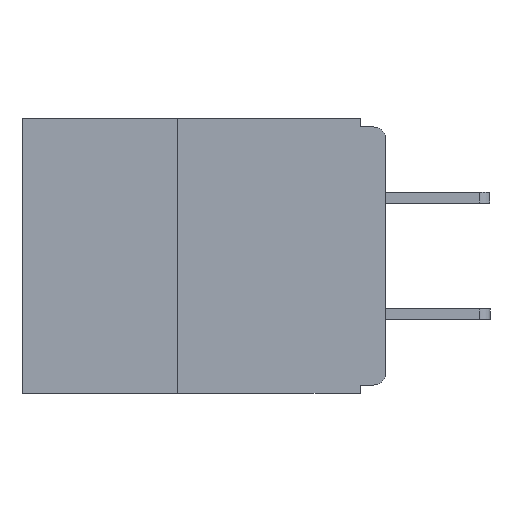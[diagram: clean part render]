
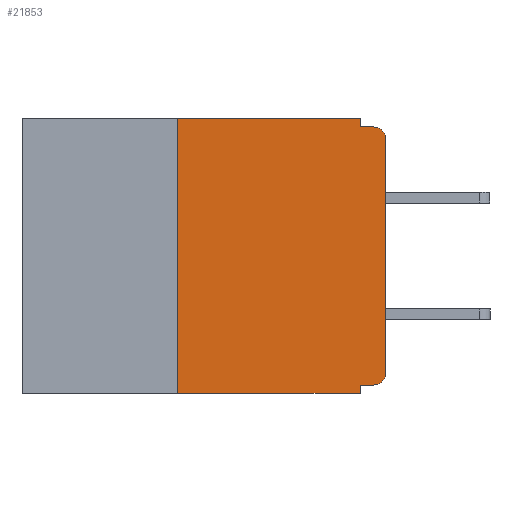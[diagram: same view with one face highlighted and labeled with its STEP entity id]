
A CAD part, left-side view. The second image highlights one B-rep face of the part: STEP entity #21853.
In plain terms, the highlighted planar face has unit normal (-1, 0, 0).
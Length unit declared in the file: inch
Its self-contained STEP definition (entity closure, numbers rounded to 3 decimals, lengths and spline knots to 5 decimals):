
#26 = DIRECTION ( 'NONE',  ( 0., 0., -1. ) ) ;
#182 = LINE ( 'NONE', #5568, #24632 ) ;
#545 = CIRCLE ( 'NONE', #4228, 0.015 ) ;
#1150 = VERTEX_POINT ( 'NONE', #28312 ) ;
#1469 = EDGE_CURVE ( 'NONE', #29636, #2069, #15435, .T. ) ;
#1866 = CARTESIAN_POINT ( 'NONE',  ( 0., 0.031, 0. ) ) ;
#1931 = LINE ( 'NONE', #22578, #26181 ) ;
#1976 = CARTESIAN_POINT ( 'NONE',  ( 0., 0.031, -0.33 ) ) ;
#2069 = VERTEX_POINT ( 'NONE', #25018 ) ;
#2097 = DIRECTION ( 'NONE',  ( 0., 0., -1. ) ) ;
#2190 = VECTOR ( 'NONE', #18975, 39.37008 ) ;
#2293 = VERTEX_POINT ( 'NONE', #10409 ) ;
#2491 = VECTOR ( 'NONE', #17809, 39.37008 ) ;
#2676 = FACE_OUTER_BOUND ( 'NONE', #25250, .T. ) ;
#2992 = ORIENTED_EDGE ( 'NONE', *, *, #18980, .T. ) ;
#3716 = LINE ( 'NONE', #15430, #27130 ) ;
#3831 = CARTESIAN_POINT ( 'NONE',  ( 0., 0.031, -0.01 ) ) ;
#4228 = AXIS2_PLACEMENT_3D ( 'NONE', #13681, #29791, #16025 ) ;
#5568 = CARTESIAN_POINT ( 'NONE',  ( 0., 0.031, 0. ) ) ;
#5928 = ORIENTED_EDGE ( 'NONE', *, *, #9402, .F. ) ;
#6290 = ORIENTED_EDGE ( 'NONE', *, *, #24210, .T. ) ;
#7360 = ORIENTED_EDGE ( 'NONE', *, *, #25891, .F. ) ;
#7469 = VERTEX_POINT ( 'NONE', #1866 ) ;
#8185 = DIRECTION ( 'NONE',  ( 0., 0., 1. ) ) ;
#8435 = AXIS2_PLACEMENT_3D ( 'NONE', #13948, #16298, #2097 ) ;
#8697 = LINE ( 'NONE', #24704, #2491 ) ;
#9402 = EDGE_CURVE ( 'NONE', #20168, #25844, #14808, .T. ) ;
#9534 = CARTESIAN_POINT ( 'NONE',  ( 0., 0.031, -0.33 ) ) ;
#10409 = CARTESIAN_POINT ( 'NONE',  ( 0., 0., -0.305 ) ) ;
#10412 = CARTESIAN_POINT ( 'NONE',  ( 0., 0.015, -0.01 ) ) ;
#10451 = LINE ( 'NONE', #9534, #16031 ) ;
#10753 = DIRECTION ( 'NONE',  ( 0., -1., 0. ) ) ;
#10789 = VERTEX_POINT ( 'NONE', #28320 ) ;
#11145 = ORIENTED_EDGE ( 'NONE', *, *, #1469, .F. ) ;
#12031 = CARTESIAN_POINT ( 'NONE',  ( 0., 0.015, -0.025 ) ) ;
#13215 = VERTEX_POINT ( 'NONE', #1976 ) ;
#13681 = CARTESIAN_POINT ( 'NONE',  ( 0., 0.015, -0.305 ) ) ;
#13945 = VERTEX_POINT ( 'NONE', #23616 ) ;
#13948 = CARTESIAN_POINT ( 'NONE',  ( 0., 0.437, 0. ) ) ;
#14240 = CARTESIAN_POINT ( 'NONE',  ( 0., 0., -0.01 ) ) ;
#14371 = CARTESIAN_POINT ( 'NONE',  ( 0., 0.015, -0.32 ) ) ;
#14409 = DIRECTION ( 'NONE',  ( 0., 0., -1. ) ) ;
#14808 = LINE ( 'NONE', #14240, #2190 ) ;
#15245 = ORIENTED_EDGE ( 'NONE', *, *, #21317, .F. ) ;
#15417 = CARTESIAN_POINT ( 'NONE',  ( 0., 0., -0.32 ) ) ;
#15430 = CARTESIAN_POINT ( 'NONE',  ( 0., 0.437, -0.33 ) ) ;
#15435 = LINE ( 'NONE', #15417, #20929 ) ;
#15629 = VECTOR ( 'NONE', #8185, 39.37008 ) ;
#16025 = DIRECTION ( 'NONE',  ( 0., 0., -1. ) ) ;
#16031 = VECTOR ( 'NONE', #26, 39.37008 ) ;
#16298 = DIRECTION ( 'NONE',  ( 1., 0., 0. ) ) ;
#17693 = CARTESIAN_POINT ( 'NONE',  ( 0., 0.25, -0.33 ) ) ;
#17809 = DIRECTION ( 'NONE',  ( 0., -1., 0. ) ) ;
#18975 = DIRECTION ( 'NONE',  ( 0., -1., 0. ) ) ;
#18980 = EDGE_CURVE ( 'NONE', #2293, #1150, #1931, .T. ) ;
#19727 = DIRECTION ( 'NONE',  ( 0., 0., -1. ) ) ;
#20168 = VERTEX_POINT ( 'NONE', #3831 ) ;
#20929 = VECTOR ( 'NONE', #27915, 39.37008 ) ;
#21317 = EDGE_CURVE ( 'NONE', #2069, #13215, #10451, .T. ) ;
#21853 = ADVANCED_FACE ( 'NONE', ( #2676 ), #27803, .F. ) ;
#22578 = CARTESIAN_POINT ( 'NONE',  ( 0., 0., 0. ) ) ;
#22857 = EDGE_CURVE ( 'NONE', #10789, #13215, #3716, .T. ) ;
#23278 = ORIENTED_EDGE ( 'NONE', *, *, #27224, .T. ) ;
#23616 = CARTESIAN_POINT ( 'NONE',  ( 0., 0.25, 0. ) ) ;
#23631 = AXIS2_PLACEMENT_3D ( 'NONE', #12031, #28232, #14409 ) ;
#24210 = EDGE_CURVE ( 'NONE', #29636, #2293, #545, .T. ) ;
#24284 = CIRCLE ( 'NONE', #23631, 0.015 ) ;
#24632 = VECTOR ( 'NONE', #19727, 39.37008 ) ;
#24691 = ORIENTED_EDGE ( 'NONE', *, *, #27399, .F. ) ;
#24704 = CARTESIAN_POINT ( 'NONE',  ( 0., 0.437, 0. ) ) ;
#25018 = CARTESIAN_POINT ( 'NONE',  ( 0., 0.031, -0.32 ) ) ;
#25250 = EDGE_LOOP ( 'NONE', ( #2992, #23278, #5928, #24691, #25399, #7360, #26820, #15245, #11145, #6290 ) ) ;
#25399 = ORIENTED_EDGE ( 'NONE', *, *, #28839, .F. ) ;
#25844 = VERTEX_POINT ( 'NONE', #10412 ) ;
#25891 = EDGE_CURVE ( 'NONE', #10789, #13945, #27900, .T. ) ;
#26181 = VECTOR ( 'NONE', #27118, 39.37008 ) ;
#26820 = ORIENTED_EDGE ( 'NONE', *, *, #22857, .T. ) ;
#27118 = DIRECTION ( 'NONE',  ( 0., 0., 1. ) ) ;
#27130 = VECTOR ( 'NONE', #10753, 39.37008 ) ;
#27224 = EDGE_CURVE ( 'NONE', #1150, #25844, #24284, .T. ) ;
#27399 = EDGE_CURVE ( 'NONE', #7469, #20168, #182, .T. ) ;
#27803 = PLANE ( 'NONE',  #8435 ) ;
#27900 = LINE ( 'NONE', #17693, #15629 ) ;
#27915 = DIRECTION ( 'NONE',  ( 0., 1., 0. ) ) ;
#28232 = DIRECTION ( 'NONE',  ( -1., 0., 0. ) ) ;
#28312 = CARTESIAN_POINT ( 'NONE',  ( 0., 0., -0.025 ) ) ;
#28320 = CARTESIAN_POINT ( 'NONE',  ( 0., 0.25, -0.33 ) ) ;
#28839 = EDGE_CURVE ( 'NONE', #13945, #7469, #8697, .T. ) ;
#29636 = VERTEX_POINT ( 'NONE', #14371 ) ;
#29791 = DIRECTION ( 'NONE',  ( -1., 0., 0. ) ) ;
